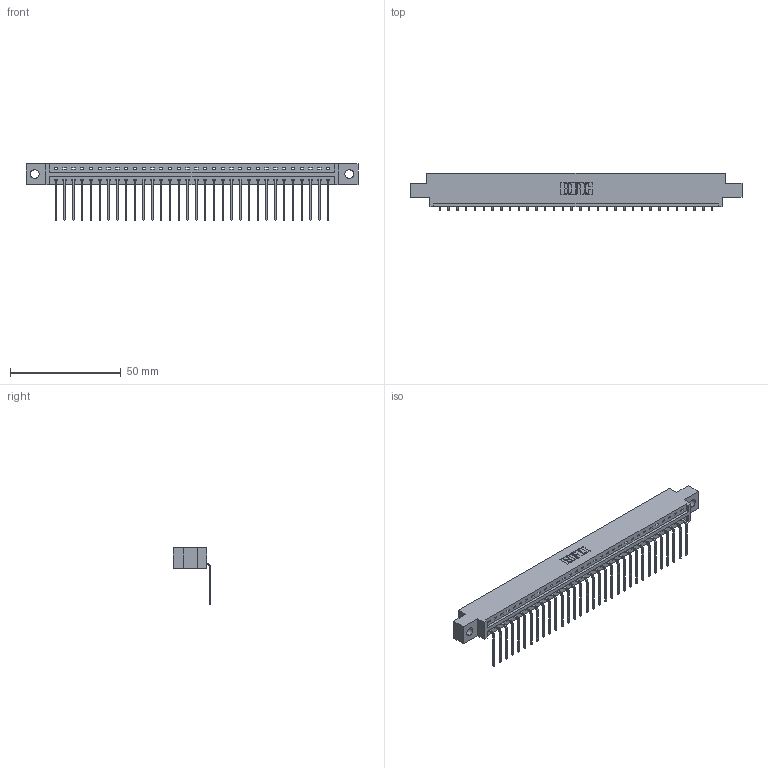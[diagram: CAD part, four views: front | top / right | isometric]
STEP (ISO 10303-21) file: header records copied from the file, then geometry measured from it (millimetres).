
FILE_DESCRIPTION (( 'STEP AP203' ), '1' );
FILE_NAME ('337-032-559-604.STEP', '2018-08-07T07:35:27', ( '' ), ( '' ), 'SwSTEP 2.0', 'SolidWorks 2016', '' );
FILE_SCHEMA (( 'CONFIG_CONTROL_DESIGN' ));
Length unit declared in the file: inch
Products named in the file (3): 337-032-559-604; 337 Part_0.170 Offset - 0.156 Dia-TH; 345-292-001_558 559 Tail - 1
Assembly tree (33 placements, depth 2):
  337-032-559-604
    337 Part_0.170 Offset - 0.156 Dia-TH
    345-292-001_558 559 Tail - 1  x32
Bounding box: 149.81 x 17.09 x 25.53 mm (x, y, z)
Volume: 15346.3 mm3; surface area: 16349.3 mm2
Topology: 33 solids, 33 shells, 2166 faces, 6531 edges, 4310 vertices
Faces by surface type: plane 1610, cylinder 556
Entity records: 25299 total; most frequent: CARTESIAN_POINT 4414, ORIENTED_EDGE 4382, DIRECTION 3735, EDGE_CURVE 2191, LINE 2063, VECTOR 2063, VERTEX_POINT 1458, AXIS2_PLACEMENT_3D 836
